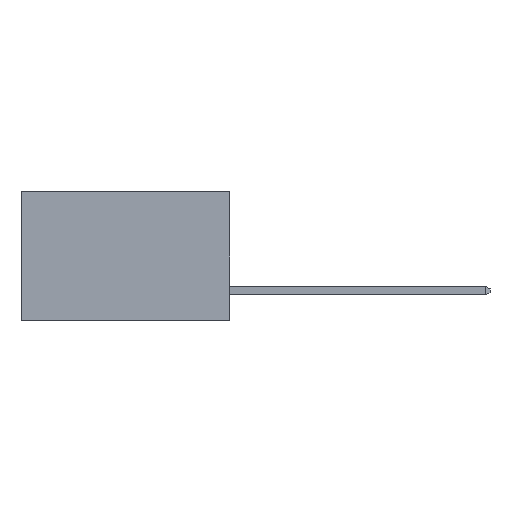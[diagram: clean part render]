
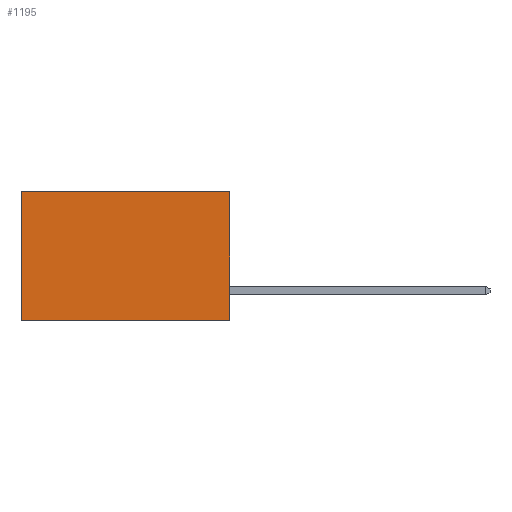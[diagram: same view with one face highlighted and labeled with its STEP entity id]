
A CAD part, left-side view. The second image highlights one B-rep face of the part: STEP entity #1195.
In plain terms, the highlighted planar face has unit normal (-1, 0, 0).
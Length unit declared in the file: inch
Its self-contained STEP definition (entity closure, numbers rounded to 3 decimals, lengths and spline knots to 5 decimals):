
#97 = LINE ( 'NONE', #10963, #1754 ) ;
#251 = DIRECTION ( 'NONE',  ( 0., 1., 0. ) ) ;
#319 = AXIS2_PLACEMENT_3D ( 'NONE', #7238, #13330, #7327 ) ;
#975 = EDGE_CURVE ( 'NONE', #3038, #8480, #1532, .T. ) ;
#1156 = CARTESIAN_POINT ( 'NONE',  ( 0.2615, 0., 0. ) ) ;
#1195 = ADVANCED_FACE ( 'NONE', ( #7139 ), #9226, .F. ) ;
#1532 = LINE ( 'NONE', #5956, #11189 ) ;
#1754 = VECTOR ( 'NONE', #13028, 39.37008 ) ;
#2706 = VECTOR ( 'NONE', #6773, 39.37008 ) ;
#3038 = VERTEX_POINT ( 'NONE', #1156 ) ;
#3148 = ORIENTED_EDGE ( 'NONE', *, *, #975, .T. ) ;
#4139 = ORIENTED_EDGE ( 'NONE', *, *, #11453, .F. ) ;
#4192 = CARTESIAN_POINT ( 'NONE',  ( 0.2615, 0.6, 0. ) ) ;
#4314 = VECTOR ( 'NONE', #251, 39.37008 ) ;
#4327 = EDGE_CURVE ( 'NONE', #3038, #10195, #7032, .T. ) ;
#5709 = ORIENTED_EDGE ( 'NONE', *, *, #4327, .F. ) ;
#5712 = ORIENTED_EDGE ( 'NONE', *, *, #11723, .T. ) ;
#5956 = CARTESIAN_POINT ( 'NONE',  ( 0.2615, 0., 0. ) ) ;
#6340 = CARTESIAN_POINT ( 'NONE',  ( 0.2615, 0., -0.37 ) ) ;
#6389 = LINE ( 'NONE', #6340, #4314 ) ;
#6773 = DIRECTION ( 'NONE',  ( 0., 0., -1. ) ) ;
#7032 = LINE ( 'NONE', #8757, #2706 ) ;
#7139 = FACE_OUTER_BOUND ( 'NONE', #10310, .T. ) ;
#7238 = CARTESIAN_POINT ( 'NONE',  ( 0.2615, 0., -0.37 ) ) ;
#7327 = DIRECTION ( 'NONE',  ( 0., 0., -1. ) ) ;
#8480 = VERTEX_POINT ( 'NONE', #4192 ) ;
#8717 = CARTESIAN_POINT ( 'NONE',  ( 0.2615, 0., -0.37 ) ) ;
#8757 = CARTESIAN_POINT ( 'NONE',  ( 0.2615, 0., -0.37 ) ) ;
#8845 = VERTEX_POINT ( 'NONE', #9652 ) ;
#9226 = PLANE ( 'NONE',  #319 ) ;
#9652 = CARTESIAN_POINT ( 'NONE',  ( 0.2615, 0.6, -0.37 ) ) ;
#10195 = VERTEX_POINT ( 'NONE', #8717 ) ;
#10310 = EDGE_LOOP ( 'NONE', ( #5712, #4139, #5709, #3148 ) ) ;
#10963 = CARTESIAN_POINT ( 'NONE',  ( 0.2615, 0.6, -0.37 ) ) ;
#11189 = VECTOR ( 'NONE', #12103, 39.37008 ) ;
#11453 = EDGE_CURVE ( 'NONE', #10195, #8845, #6389, .T. ) ;
#11723 = EDGE_CURVE ( 'NONE', #8480, #8845, #97, .T. ) ;
#12103 = DIRECTION ( 'NONE',  ( 0., 1., 0. ) ) ;
#13028 = DIRECTION ( 'NONE',  ( 0., 0., -1. ) ) ;
#13330 = DIRECTION ( 'NONE',  ( 1., 0., 0. ) ) ;
